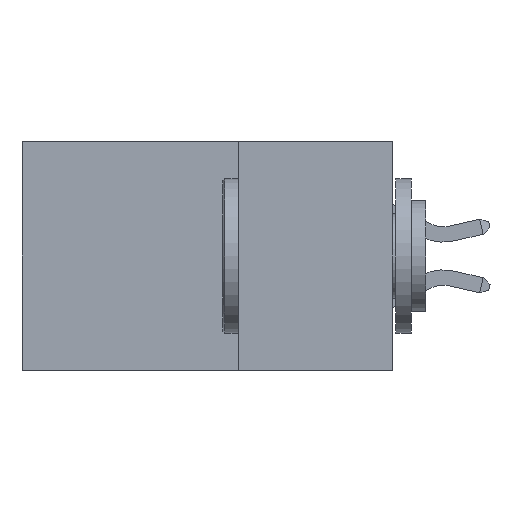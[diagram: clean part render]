
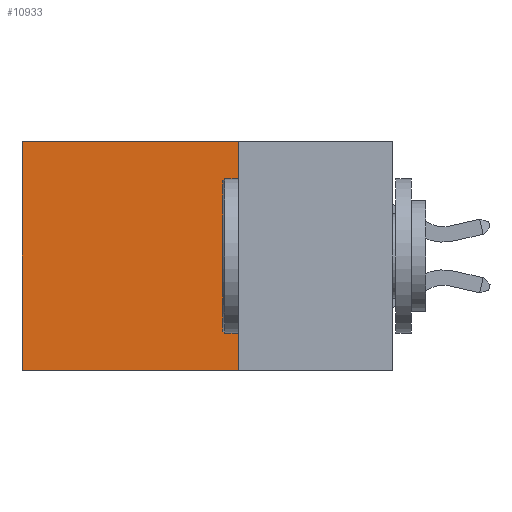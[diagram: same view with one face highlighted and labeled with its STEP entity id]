
A CAD part, left-side view. The second image highlights one B-rep face of the part: STEP entity #10933.
In plain terms, the highlighted planar face has unit normal (-1, 0, 0).
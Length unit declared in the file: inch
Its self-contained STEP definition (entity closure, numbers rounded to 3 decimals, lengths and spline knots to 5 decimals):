
#298 = CARTESIAN_POINT ( 'NONE',  ( 0.2875, 0.25, 0. ) ) ;
#434 = VECTOR ( 'NONE', #6031, 39.37008 ) ;
#472 = CARTESIAN_POINT ( 'NONE',  ( 0.2875, 0.25, 0. ) ) ;
#570 = VERTEX_POINT ( 'NONE', #10869 ) ;
#2066 = DIRECTION ( 'NONE',  ( 0., 1., 0. ) ) ;
#2282 = VERTEX_POINT ( 'NONE', #3501 ) ;
#2848 = CARTESIAN_POINT ( 'NONE',  ( 0.2875, 0.25, -0.37 ) ) ;
#2964 = CARTESIAN_POINT ( 'NONE',  ( 0.2875, 0.25, 0. ) ) ;
#3215 = CARTESIAN_POINT ( 'NONE',  ( 0.2875, 0.25, -0.37 ) ) ;
#3334 = FACE_OUTER_BOUND ( 'NONE', #5463, .T. ) ;
#3408 = CARTESIAN_POINT ( 'NONE',  ( 0.2875, 0.6, 0. ) ) ;
#3501 = CARTESIAN_POINT ( 'NONE',  ( 0.2875, 0.6, 0. ) ) ;
#3576 = EDGE_CURVE ( 'NONE', #4470, #570, #3600, .T. ) ;
#3600 = LINE ( 'NONE', #2848, #3892 ) ;
#3868 = ORIENTED_EDGE ( 'NONE', *, *, #3576, .F. ) ;
#3892 = VECTOR ( 'NONE', #2066, 39.37008 ) ;
#4470 = VERTEX_POINT ( 'NONE', #3215 ) ;
#4524 = ORIENTED_EDGE ( 'NONE', *, *, #8534, .T. ) ;
#4586 = ORIENTED_EDGE ( 'NONE', *, *, #9386, .F. ) ;
#4618 = DIRECTION ( 'NONE',  ( 0., 0., -1. ) ) ;
#4632 = AXIS2_PLACEMENT_3D ( 'NONE', #7114, #5528, #4618 ) ;
#5383 = LINE ( 'NONE', #472, #10380 ) ;
#5463 = EDGE_LOOP ( 'NONE', ( #4524, #3868, #4586, #7660 ) ) ;
#5528 = DIRECTION ( 'NONE',  ( 1., 0., 0. ) ) ;
#6031 = DIRECTION ( 'NONE',  ( 0., 0., -1. ) ) ;
#6196 = DIRECTION ( 'NONE',  ( 0., 1., 0. ) ) ;
#6787 = LINE ( 'NONE', #298, #6887 ) ;
#6887 = VECTOR ( 'NONE', #6196, 39.37008 ) ;
#7099 = EDGE_CURVE ( 'NONE', #10354, #2282, #6787, .T. ) ;
#7114 = CARTESIAN_POINT ( 'NONE',  ( 0.2875, 0.25, 0. ) ) ;
#7660 = ORIENTED_EDGE ( 'NONE', *, *, #7099, .T. ) ;
#8534 = EDGE_CURVE ( 'NONE', #2282, #570, #8745, .T. ) ;
#8745 = LINE ( 'NONE', #3408, #434 ) ;
#8838 = PLANE ( 'NONE',  #4632 ) ;
#9386 = EDGE_CURVE ( 'NONE', #10354, #4470, #5383, .T. ) ;
#10354 = VERTEX_POINT ( 'NONE', #2964 ) ;
#10380 = VECTOR ( 'NONE', #10830, 39.37008 ) ;
#10830 = DIRECTION ( 'NONE',  ( 0., 0., -1. ) ) ;
#10869 = CARTESIAN_POINT ( 'NONE',  ( 0.2875, 0.6, -0.37 ) ) ;
#10933 = ADVANCED_FACE ( 'NONE', ( #3334 ), #8838, .F. ) ;
